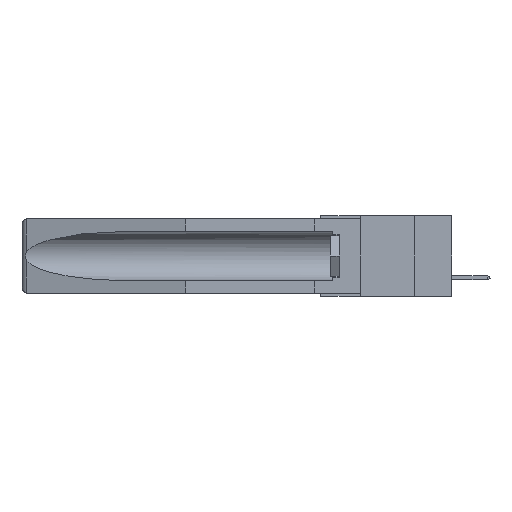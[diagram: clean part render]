
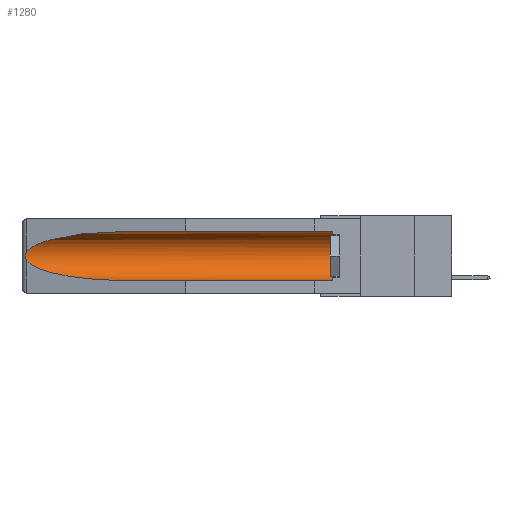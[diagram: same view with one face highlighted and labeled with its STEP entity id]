
A CAD part, left-side view. The second image highlights one B-rep face of the part: STEP entity #1280.
In plain terms, the highlighted cylindrical face has radius 2.857 mm (diameter 5.715 mm), a partial arc.
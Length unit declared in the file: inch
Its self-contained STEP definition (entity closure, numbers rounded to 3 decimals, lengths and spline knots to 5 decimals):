
#286 = CYLINDRICAL_SURFACE ( 'NONE', #435, 0.1125 ) ;
#435 = AXIS2_PLACEMENT_3D ( 'NONE', #12729, #3551, #20037 ) ;
#1280 = ADVANCED_FACE ( 'NONE', ( #15928 ), #286, .F. ) ;
#1299 = CARTESIAN_POINT ( 'NONE',  ( 0.21114, 1.30732, -0.284 ) ) ;
#1554 = CARTESIAN_POINT ( 'NONE',  ( 0.155, -0.30754, -0.284 ) ) ;
#1600 = EDGE_LOOP ( 'NONE', ( #17986, #13267, #7261, #20412, #18024, #4251 ) ) ;
#2100 = CARTESIAN_POINT ( 'NONE',  ( 0.26537, 1.52718, -0.14972 ) ) ;
#3021 = EDGE_CURVE ( 'NONE', #5359, #3280, #6143, .T. ) ;
#3049 = LINE ( 'NONE', #4227, #21465 ) ;
#3052 = CARTESIAN_POINT ( 'NONE',  ( 0.155, 1.07973, -0.284 ) ) ;
#3280 = VERTEX_POINT ( 'NONE', #16733 ) ;
#3354 = CARTESIAN_POINT ( 'NONE',  ( 0.26597, 1.5296, -0.19026 ) ) ;
#3551 = DIRECTION ( 'NONE',  ( 0., 1., 0. ) ) ;
#3790 = EDGE_CURVE ( 'NONE', #6542, #20142, #14974, .T. ) ;
#4058 = CARTESIAN_POINT ( 'NONE',  ( 0.2675, 1.53308, -0.17534 ) ) ;
#4227 = CARTESIAN_POINT ( 'NONE',  ( 0.155, -0.30754, -0.059 ) ) ;
#4251 = ORIENTED_EDGE ( 'NONE', *, *, #6012, .T. ) ;
#4641 = CARTESIAN_POINT ( 'NONE',  ( 0.155, 1.07973, -0.284 ) ) ;
#4776 = VECTOR ( 'NONE', #18268, 39.37008 ) ;
#5359 = VERTEX_POINT ( 'NONE', #20650 ) ;
#5790 = CARTESIAN_POINT ( 'NONE',  ( 0.26597, 1.52961, -0.15275 ) ) ;
#6012 = EDGE_CURVE ( 'NONE', #3280, #6542, #3049, .T. ) ;
#6143 = CIRCLE ( 'NONE', #21088, 0.1125 ) ;
#6542 = VERTEX_POINT ( 'NONE', #19520 ) ;
#7261 = ORIENTED_EDGE ( 'NONE', *, *, #9503, .T. ) ;
#7372 = CARTESIAN_POINT ( 'NONE',  ( 0.26654, 1.53092, -0.15636 ) ) ;
#7661 =( BOUNDED_CURVE ( )  B_SPLINE_CURVE ( 3, ( #12058, #10231, #1299, #3052 ),
 .UNSPECIFIED., .F., .F. ) 
 B_SPLINE_CURVE_WITH_KNOTS ( ( 4, 4 ),
 ( 0.1948, 1.5708 ),
 .UNSPECIFIED. ) 
 CURVE ( )  GEOMETRIC_REPRESENTATION_ITEM ( )  RATIONAL_B_SPLINE_CURVE ( ( 1., 0.848, 0.848, 1. ) ) 
 REPRESENTATION_ITEM ( '' )  );
#7970 = B_SPLINE_CURVE_WITH_KNOTS ( 'NONE', 3,
 ( #16790, #5790, #7372, #22114, #14940, #4058, #12864, #21339, #3354, #19460 ),
 .UNSPECIFIED., .F., .F.,
 ( 4, 2, 2, 2, 4 ),
 ( 0., 0.00029, 0.00058, 0.00087, 0.00117 ),
 .UNSPECIFIED. ) ;
#8656 = CARTESIAN_POINT ( 'NONE',  ( 0.155, 1.07973, -0.059 ) ) ;
#9503 = EDGE_CURVE ( 'NONE', #14452, #14372, #7661, .T. ) ;
#10231 = CARTESIAN_POINT ( 'NONE',  ( 0.25451, 1.48313, -0.24835 ) ) ;
#11071 = EDGE_CURVE ( 'NONE', #5359, #14372, #17568, .T. ) ;
#12058 = CARTESIAN_POINT ( 'NONE',  ( 0.26537, 1.52718, -0.19328 ) ) ;
#12509 = DIRECTION ( 'NONE',  ( 0., 0., 1. ) ) ;
#12640 = CARTESIAN_POINT ( 'NONE',  ( 0.21114, 1.30732, -0.059 ) ) ;
#12729 = CARTESIAN_POINT ( 'NONE',  ( 0.155, -0.30754, -0.1715 ) ) ;
#12864 = CARTESIAN_POINT ( 'NONE',  ( 0.2673, 1.53269, -0.17917 ) ) ;
#12942 = CARTESIAN_POINT ( 'NONE',  ( 0.26537, 1.52718, -0.19328 ) ) ;
#13267 = ORIENTED_EDGE ( 'NONE', *, *, #17812, .T. ) ;
#13273 = CARTESIAN_POINT ( 'NONE',  ( 0.26537, 1.52718, -0.14972 ) ) ;
#14372 = VERTEX_POINT ( 'NONE', #4641 ) ;
#14452 = VERTEX_POINT ( 'NONE', #12942 ) ;
#14940 = CARTESIAN_POINT ( 'NONE',  ( 0.2675, 1.53308, -0.16763 ) ) ;
#14974 =( BOUNDED_CURVE ( )  B_SPLINE_CURVE ( 3, ( #8656, #12640, #16007, #2100 ),
 .UNSPECIFIED., .F., .F. ) 
 B_SPLINE_CURVE_WITH_KNOTS ( ( 4, 4 ),
 ( 4.71239, 6.08839 ),
 .UNSPECIFIED. ) 
 CURVE ( )  GEOMETRIC_REPRESENTATION_ITEM ( )  RATIONAL_B_SPLINE_CURVE ( ( 1., 0.848, 0.848, 1. ) ) 
 REPRESENTATION_ITEM ( '' )  );
#15928 = FACE_OUTER_BOUND ( 'NONE', #1600, .T. ) ;
#16007 = CARTESIAN_POINT ( 'NONE',  ( 0.25451, 1.48313, -0.09465 ) ) ;
#16733 = CARTESIAN_POINT ( 'NONE',  ( 0.155, 0.126, -0.059 ) ) ;
#16790 = CARTESIAN_POINT ( 'NONE',  ( 0.26537, 1.52718, -0.14972 ) ) ;
#17568 = LINE ( 'NONE', #1554, #4776 ) ;
#17812 = EDGE_CURVE ( 'NONE', #20142, #14452, #7970, .T. ) ;
#17928 = DIRECTION ( 'NONE',  ( 0., -1., 0. ) ) ;
#17986 = ORIENTED_EDGE ( 'NONE', *, *, #3790, .T. ) ;
#18024 = ORIENTED_EDGE ( 'NONE', *, *, #3021, .T. ) ;
#18268 = DIRECTION ( 'NONE',  ( 0., 1., 0. ) ) ;
#19460 = CARTESIAN_POINT ( 'NONE',  ( 0.26537, 1.52718, -0.19328 ) ) ;
#19520 = CARTESIAN_POINT ( 'NONE',  ( 0.155, 1.07973, -0.059 ) ) ;
#20037 = DIRECTION ( 'NONE',  ( 0., 0., 1. ) ) ;
#20142 = VERTEX_POINT ( 'NONE', #13273 ) ;
#20412 = ORIENTED_EDGE ( 'NONE', *, *, #11071, .F. ) ;
#20650 = CARTESIAN_POINT ( 'NONE',  ( 0.155, 0.126, -0.284 ) ) ;
#21088 = AXIS2_PLACEMENT_3D ( 'NONE', #23120, #17928, #12509 ) ;
#21339 = CARTESIAN_POINT ( 'NONE',  ( 0.26655, 1.53094, -0.18657 ) ) ;
#21465 = VECTOR ( 'NONE', #22361, 39.37008 ) ;
#22114 = CARTESIAN_POINT ( 'NONE',  ( 0.2673, 1.5327, -0.16383 ) ) ;
#22361 = DIRECTION ( 'NONE',  ( 0., 1., 0. ) ) ;
#23120 = CARTESIAN_POINT ( 'NONE',  ( 0.155, 0.126, -0.1715 ) ) ;
